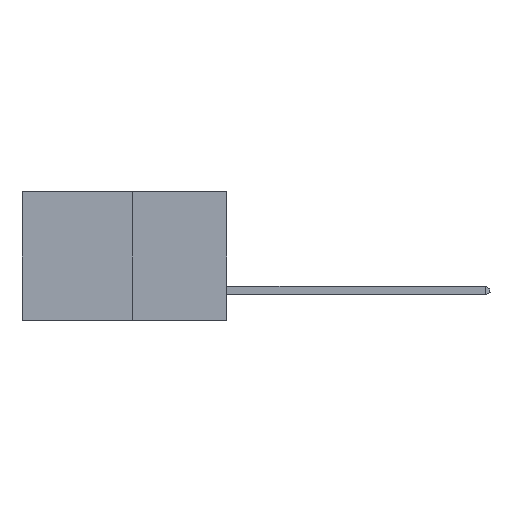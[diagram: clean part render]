
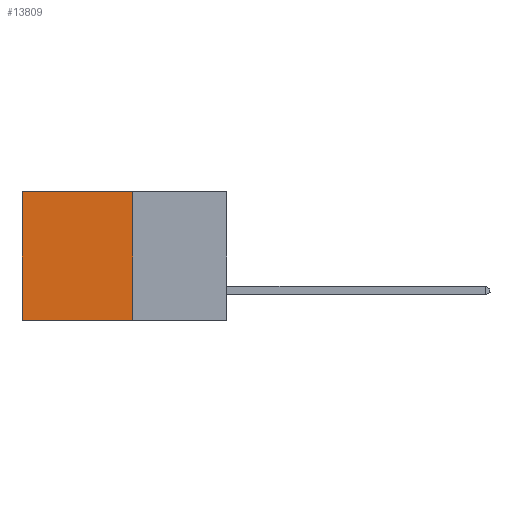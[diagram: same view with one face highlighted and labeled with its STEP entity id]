
A CAD part, left-side view. The second image highlights one B-rep face of the part: STEP entity #13809.
In plain terms, the highlighted planar face has unit normal (-1, 0, 0).
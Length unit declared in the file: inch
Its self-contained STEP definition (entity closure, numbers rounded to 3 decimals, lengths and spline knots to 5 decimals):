
#364 = EDGE_CURVE ( 'NONE', #3061, #1550, #15289, .T. ) ;
#843 = EDGE_CURVE ( 'NONE', #18501, #3061, #15043, .T. ) ;
#906 = CARTESIAN_POINT ( 'NONE',  ( 0.277, 0.59, 0. ) ) ;
#1550 = VERTEX_POINT ( 'NONE', #2390 ) ;
#1850 = EDGE_CURVE ( 'NONE', #18501, #8509, #20343, .T. ) ;
#2295 = ORIENTED_EDGE ( 'NONE', *, *, #364, .T. ) ;
#2390 = CARTESIAN_POINT ( 'NONE',  ( 0.277, 0.59, -0.37 ) ) ;
#2492 = ORIENTED_EDGE ( 'NONE', *, *, #9564, .F. ) ;
#2516 = ORIENTED_EDGE ( 'NONE', *, *, #1850, .F. ) ;
#2719 = ORIENTED_EDGE ( 'NONE', *, *, #843, .T. ) ;
#3061 = VERTEX_POINT ( 'NONE', #906 ) ;
#4476 = VECTOR ( 'NONE', #16282, 39.37008 ) ;
#4811 = CARTESIAN_POINT ( 'NONE',  ( 0.277, 0.59, -0.37 ) ) ;
#5110 = CARTESIAN_POINT ( 'NONE',  ( 0.277, 0.27, -0.37 ) ) ;
#6630 = VECTOR ( 'NONE', #15780, 39.37008 ) ;
#8030 = DIRECTION ( 'NONE',  ( 0., 0., -1. ) ) ;
#8340 = CARTESIAN_POINT ( 'NONE',  ( 0.277, 0.27, -0.37 ) ) ;
#8509 = VERTEX_POINT ( 'NONE', #10113 ) ;
#9564 = EDGE_CURVE ( 'NONE', #8509, #1550, #12468, .T. ) ;
#9915 = DIRECTION ( 'NONE',  ( 0., 0., -1. ) ) ;
#10113 = CARTESIAN_POINT ( 'NONE',  ( 0.277, 0.27, -0.37 ) ) ;
#12468 = LINE ( 'NONE', #8340, #4476 ) ;
#13809 = ADVANCED_FACE ( 'NONE', ( #17201 ), #16264, .F. ) ;
#15043 = LINE ( 'NONE', #18287, #6630 ) ;
#15289 = LINE ( 'NONE', #4811, #18941 ) ;
#15780 = DIRECTION ( 'NONE',  ( 0., 1., 0. ) ) ;
#15923 = EDGE_LOOP ( 'NONE', ( #2295, #2492, #2516, #2719 ) ) ;
#16263 = VECTOR ( 'NONE', #17687, 39.37008 ) ;
#16264 = PLANE ( 'NONE',  #16493 ) ;
#16282 = DIRECTION ( 'NONE',  ( 0., 1., 0. ) ) ;
#16493 = AXIS2_PLACEMENT_3D ( 'NONE', #5110, #19353, #9915 ) ;
#16671 = CARTESIAN_POINT ( 'NONE',  ( 0.277, 0.27, -0.37 ) ) ;
#17201 = FACE_OUTER_BOUND ( 'NONE', #15923, .T. ) ;
#17687 = DIRECTION ( 'NONE',  ( 0., 0., -1. ) ) ;
#18287 = CARTESIAN_POINT ( 'NONE',  ( 0.277, 0.27, 0. ) ) ;
#18501 = VERTEX_POINT ( 'NONE', #19566 ) ;
#18941 = VECTOR ( 'NONE', #8030, 39.37008 ) ;
#19353 = DIRECTION ( 'NONE',  ( 1., 0., 0. ) ) ;
#19566 = CARTESIAN_POINT ( 'NONE',  ( 0.277, 0.27, 0. ) ) ;
#20343 = LINE ( 'NONE', #16671, #16263 ) ;
